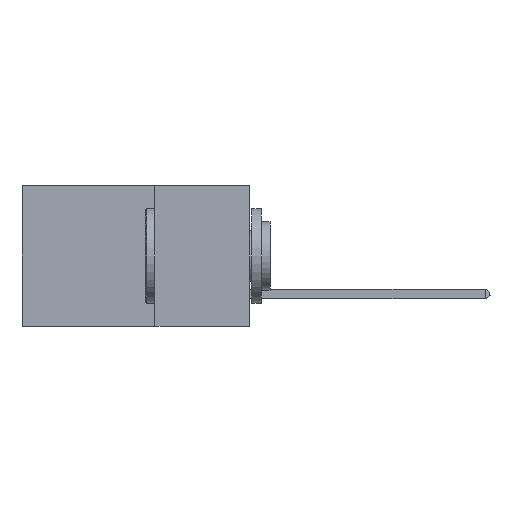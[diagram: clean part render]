
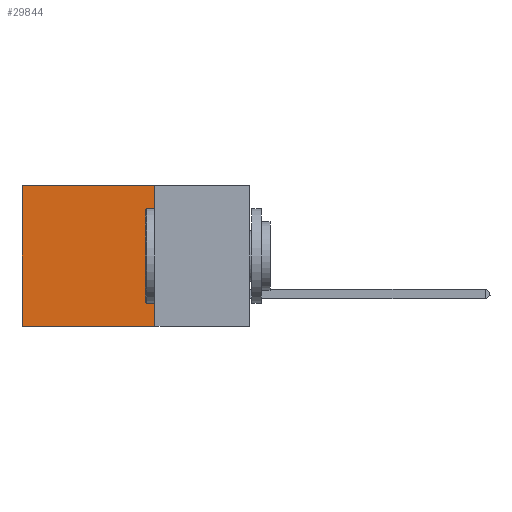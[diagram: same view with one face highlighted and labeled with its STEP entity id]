
A CAD part, left-side view. The second image highlights one B-rep face of the part: STEP entity #29844.
In plain terms, the highlighted planar face has unit normal (-1, 0, 0).
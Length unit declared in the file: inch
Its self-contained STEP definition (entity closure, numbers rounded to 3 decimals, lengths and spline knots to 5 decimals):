
#177 = EDGE_CURVE ( 'NONE', #28965, #23390, #25154, .T. ) ;
#1974 = DIRECTION ( 'NONE',  ( 0., 0., -1. ) ) ;
#3246 = CARTESIAN_POINT ( 'NONE',  ( 0.2875, 0.25, 0. ) ) ;
#3496 = VECTOR ( 'NONE', #8081, 39.37008 ) ;
#4603 = VECTOR ( 'NONE', #18144, 39.37008 ) ;
#6125 = FACE_OUTER_BOUND ( 'NONE', #10297, .T. ) ;
#7576 = ORIENTED_EDGE ( 'NONE', *, *, #27315, .F. ) ;
#7878 = DIRECTION ( 'NONE',  ( 0., 1., 0. ) ) ;
#8081 = DIRECTION ( 'NONE',  ( 0., 1., 0. ) ) ;
#8708 = LINE ( 'NONE', #3246, #28116 ) ;
#8777 = VERTEX_POINT ( 'NONE', #28165 ) ;
#9554 = CARTESIAN_POINT ( 'NONE',  ( 0.2875, 0.25, -0.37 ) ) ;
#10283 = DIRECTION ( 'NONE',  ( 0., 0., -1. ) ) ;
#10297 = EDGE_LOOP ( 'NONE', ( #16453, #22602, #7576, #16582 ) ) ;
#10675 = EDGE_CURVE ( 'NONE', #8777, #25776, #20543, .T. ) ;
#11807 = EDGE_CURVE ( 'NONE', #25776, #23390, #27777, .T. ) ;
#12278 = CARTESIAN_POINT ( 'NONE',  ( 0.2875, 0.25, -0.37 ) ) ;
#15589 = CARTESIAN_POINT ( 'NONE',  ( 0.2875, 0.25, 0. ) ) ;
#16453 = ORIENTED_EDGE ( 'NONE', *, *, #11807, .T. ) ;
#16521 = CARTESIAN_POINT ( 'NONE',  ( 0.2875, 0.6, 0. ) ) ;
#16582 = ORIENTED_EDGE ( 'NONE', *, *, #10675, .T. ) ;
#16998 = CARTESIAN_POINT ( 'NONE',  ( 0.2875, 0.25, 0. ) ) ;
#17101 = AXIS2_PLACEMENT_3D ( 'NONE', #15589, #18178, #1974 ) ;
#18144 = DIRECTION ( 'NONE',  ( 0., 0., -1. ) ) ;
#18178 = DIRECTION ( 'NONE',  ( 1., 0., 0. ) ) ;
#20543 = LINE ( 'NONE', #16998, #28244 ) ;
#22602 = ORIENTED_EDGE ( 'NONE', *, *, #177, .F. ) ;
#23390 = VERTEX_POINT ( 'NONE', #23433 ) ;
#23433 = CARTESIAN_POINT ( 'NONE',  ( 0.2875, 0.6, -0.37 ) ) ;
#25154 = LINE ( 'NONE', #12278, #3496 ) ;
#25776 = VERTEX_POINT ( 'NONE', #16521 ) ;
#27315 = EDGE_CURVE ( 'NONE', #8777, #28965, #8708, .T. ) ;
#27430 = PLANE ( 'NONE',  #17101 ) ;
#27709 = CARTESIAN_POINT ( 'NONE',  ( 0.2875, 0.6, 0. ) ) ;
#27777 = LINE ( 'NONE', #27709, #4603 ) ;
#28116 = VECTOR ( 'NONE', #10283, 39.37008 ) ;
#28165 = CARTESIAN_POINT ( 'NONE',  ( 0.2875, 0.25, 0. ) ) ;
#28244 = VECTOR ( 'NONE', #7878, 39.37008 ) ;
#28965 = VERTEX_POINT ( 'NONE', #9554 ) ;
#29844 = ADVANCED_FACE ( 'NONE', ( #6125 ), #27430, .F. ) ;
